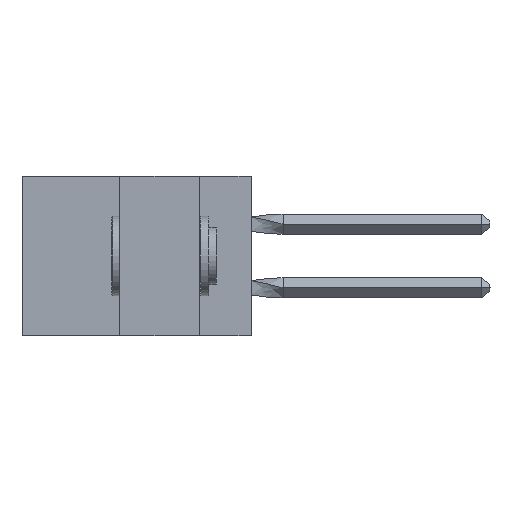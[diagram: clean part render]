
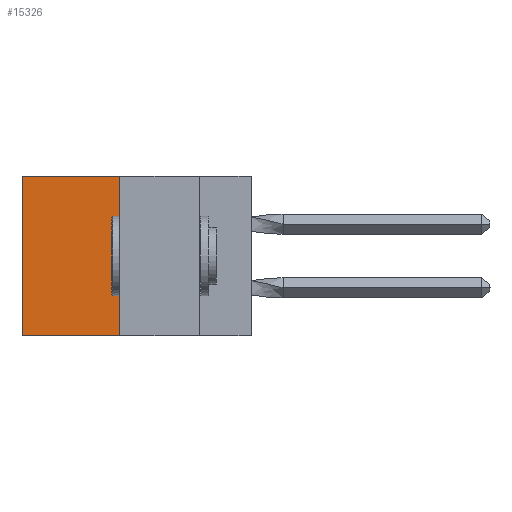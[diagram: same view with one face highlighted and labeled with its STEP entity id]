
A CAD part, left-side view. The second image highlights one B-rep face of the part: STEP entity #15326.
In plain terms, the highlighted planar face has unit normal (-1, 0, 0).
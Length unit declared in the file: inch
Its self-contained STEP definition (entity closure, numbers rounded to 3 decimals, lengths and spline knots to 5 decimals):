
#290 = CARTESIAN_POINT ( 'NONE',  ( 0.305, 0.72, -0.5 ) ) ;
#2084 = DIRECTION ( 'NONE',  ( 1., 0., 0. ) ) ;
#2097 = VERTEX_POINT ( 'NONE', #9849 ) ;
#2359 = LINE ( 'NONE', #5848, #5875 ) ;
#2950 = FACE_OUTER_BOUND ( 'NONE', #20346, .T. ) ;
#3746 = DIRECTION ( 'NONE',  ( 0., 1., 0. ) ) ;
#4223 = VECTOR ( 'NONE', #16062, 39.37008 ) ;
#4436 = ORIENTED_EDGE ( 'NONE', *, *, #10886, .F. ) ;
#5394 = CARTESIAN_POINT ( 'NONE',  ( 0.305, 0.413, -0.5 ) ) ;
#5438 = LINE ( 'NONE', #19886, #6451 ) ;
#5848 = CARTESIAN_POINT ( 'NONE',  ( 0.305, 0.413, -0.5 ) ) ;
#5875 = VECTOR ( 'NONE', #18735, 39.37008 ) ;
#6440 = VERTEX_POINT ( 'NONE', #7335 ) ;
#6451 = VECTOR ( 'NONE', #3746, 39.37008 ) ;
#7311 = VECTOR ( 'NONE', #12150, 39.37008 ) ;
#7335 = CARTESIAN_POINT ( 'NONE',  ( 0.305, 0.72, 0. ) ) ;
#7515 = EDGE_CURVE ( 'NONE', #2097, #6440, #5438, .T. ) ;
#9849 = CARTESIAN_POINT ( 'NONE',  ( 0.305, 0.413, 0. ) ) ;
#10269 = PLANE ( 'NONE',  #20328 ) ;
#10886 = EDGE_CURVE ( 'NONE', #14725, #14605, #2359, .T. ) ;
#12150 = DIRECTION ( 'NONE',  ( 0., 0., -1. ) ) ;
#12748 = CARTESIAN_POINT ( 'NONE',  ( 0.305, 0.413, -0.5 ) ) ;
#12759 = LINE ( 'NONE', #290, #4223 ) ;
#12816 = LINE ( 'NONE', #5394, #7311 ) ;
#14605 = VERTEX_POINT ( 'NONE', #15745 ) ;
#14725 = VERTEX_POINT ( 'NONE', #12748 ) ;
#14838 = ORIENTED_EDGE ( 'NONE', *, *, #17676, .F. ) ;
#14987 = EDGE_CURVE ( 'NONE', #6440, #14605, #12759, .T. ) ;
#15052 = DIRECTION ( 'NONE',  ( 0., 0., -1. ) ) ;
#15326 = ADVANCED_FACE ( 'NONE', ( #2950 ), #10269, .F. ) ;
#15480 = ORIENTED_EDGE ( 'NONE', *, *, #7515, .T. ) ;
#15508 = ORIENTED_EDGE ( 'NONE', *, *, #14987, .T. ) ;
#15745 = CARTESIAN_POINT ( 'NONE',  ( 0.305, 0.72, -0.5 ) ) ;
#16062 = DIRECTION ( 'NONE',  ( 0., 0., -1. ) ) ;
#17676 = EDGE_CURVE ( 'NONE', #2097, #14725, #12816, .T. ) ;
#18735 = DIRECTION ( 'NONE',  ( 0., 1., 0. ) ) ;
#19886 = CARTESIAN_POINT ( 'NONE',  ( 0.305, 0.413, 0. ) ) ;
#19927 = CARTESIAN_POINT ( 'NONE',  ( 0.305, 0.413, -0.5 ) ) ;
#20328 = AXIS2_PLACEMENT_3D ( 'NONE', #19927, #2084, #15052 ) ;
#20346 = EDGE_LOOP ( 'NONE', ( #15508, #4436, #14838, #15480 ) ) ;
